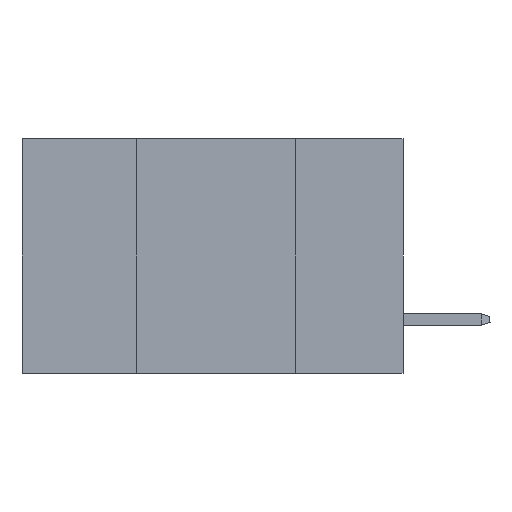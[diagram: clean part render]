
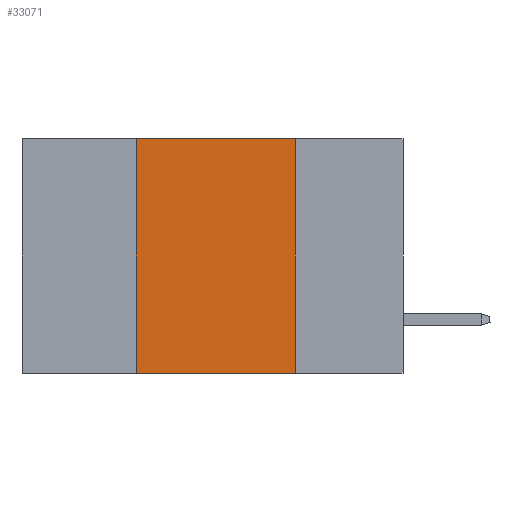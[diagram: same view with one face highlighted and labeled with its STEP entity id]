
A CAD part, left-side view. The second image highlights one B-rep face of the part: STEP entity #33071.
In plain terms, the highlighted planar face has unit normal (-1, 0, 0).
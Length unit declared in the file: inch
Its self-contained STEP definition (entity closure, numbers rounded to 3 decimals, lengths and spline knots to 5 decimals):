
#1624 = VERTEX_POINT ( 'NONE', #7223 ) ;
#4362 = CARTESIAN_POINT ( 'NONE',  ( 0., 0.17, 0. ) ) ;
#4423 = AXIS2_PLACEMENT_3D ( 'NONE', #19670, #15433, #23132 ) ;
#4545 = EDGE_LOOP ( 'NONE', ( #21720, #43798, #37160, #5528 ) ) ;
#5528 = ORIENTED_EDGE ( 'NONE', *, *, #37723, .T. ) ;
#5755 = EDGE_CURVE ( 'NONE', #30891, #1624, #12383, .T. ) ;
#6624 = VERTEX_POINT ( 'NONE', #7789 ) ;
#7223 = CARTESIAN_POINT ( 'NONE',  ( 0., 0.42, 0. ) ) ;
#7789 = CARTESIAN_POINT ( 'NONE',  ( 0., 0.17, -0.37 ) ) ;
#7969 = PLANE ( 'NONE',  #4423 ) ;
#12383 = LINE ( 'NONE', #42676, #13385 ) ;
#13385 = VECTOR ( 'NONE', #23825, 39.37008 ) ;
#13605 = EDGE_CURVE ( 'NONE', #1624, #26112, #33828, .T. ) ;
#15433 = DIRECTION ( 'NONE',  ( 1., 0., 0. ) ) ;
#16290 = LINE ( 'NONE', #4362, #21170 ) ;
#18417 = DIRECTION ( 'NONE',  ( 0., -1., 0. ) ) ;
#18649 = DIRECTION ( 'NONE',  ( 0., -1., 0. ) ) ;
#19670 = CARTESIAN_POINT ( 'NONE',  ( 0., 0.6, 0. ) ) ;
#21170 = VECTOR ( 'NONE', #23767, 39.37008 ) ;
#21720 = ORIENTED_EDGE ( 'NONE', *, *, #32145, .F. ) ;
#23132 = DIRECTION ( 'NONE',  ( 0., 0., -1. ) ) ;
#23767 = DIRECTION ( 'NONE',  ( 0., 0., -1. ) ) ;
#23825 = DIRECTION ( 'NONE',  ( 0., 0., 1. ) ) ;
#26112 = VERTEX_POINT ( 'NONE', #47706 ) ;
#30891 = VERTEX_POINT ( 'NONE', #44830 ) ;
#30963 = VECTOR ( 'NONE', #18649, 39.37008 ) ;
#32100 = VECTOR ( 'NONE', #18417, 39.37008 ) ;
#32145 = EDGE_CURVE ( 'NONE', #26112, #6624, #16290, .T. ) ;
#33071 = ADVANCED_FACE ( 'NONE', ( #41998 ), #7969, .F. ) ;
#33828 = LINE ( 'NONE', #48947, #32100 ) ;
#37160 = ORIENTED_EDGE ( 'NONE', *, *, #5755, .F. ) ;
#37494 = CARTESIAN_POINT ( 'NONE',  ( 0., 0.6, -0.37 ) ) ;
#37723 = EDGE_CURVE ( 'NONE', #30891, #6624, #40725, .T. ) ;
#40725 = LINE ( 'NONE', #37494, #30963 ) ;
#41998 = FACE_OUTER_BOUND ( 'NONE', #4545, .T. ) ;
#42676 = CARTESIAN_POINT ( 'NONE',  ( 0., 0.42, 0. ) ) ;
#43798 = ORIENTED_EDGE ( 'NONE', *, *, #13605, .F. ) ;
#44830 = CARTESIAN_POINT ( 'NONE',  ( 0., 0.42, -0.37 ) ) ;
#47706 = CARTESIAN_POINT ( 'NONE',  ( 0., 0.17, 0. ) ) ;
#48947 = CARTESIAN_POINT ( 'NONE',  ( 0., 0.6, 0. ) ) ;
